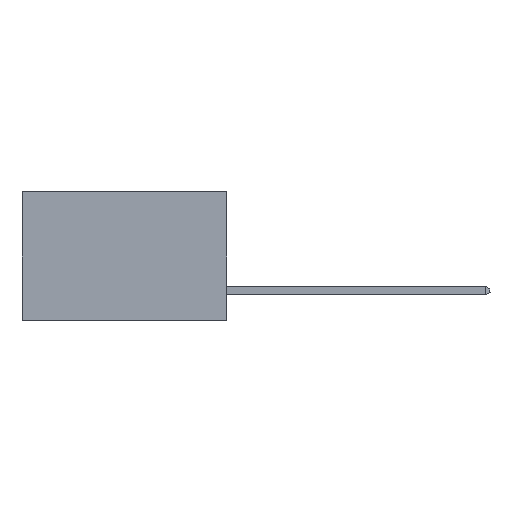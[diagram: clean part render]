
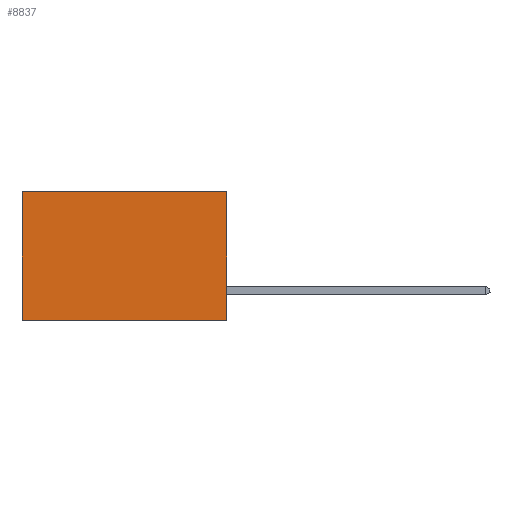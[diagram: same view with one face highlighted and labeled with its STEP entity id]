
A CAD part, left-side view. The second image highlights one B-rep face of the part: STEP entity #8837.
In plain terms, the highlighted planar face has unit normal (-1, 0, 0).
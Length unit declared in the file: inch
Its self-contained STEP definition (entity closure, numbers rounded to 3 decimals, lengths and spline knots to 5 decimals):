
#177 = VECTOR ( 'NONE', #7763, 39.37008 ) ;
#403 = LINE ( 'NONE', #4517, #2275 ) ;
#444 = VECTOR ( 'NONE', #3539, 39.37008 ) ;
#995 = CARTESIAN_POINT ( 'NONE',  ( 0.277, 0., -0.37 ) ) ;
#1180 = ORIENTED_EDGE ( 'NONE', *, *, #9418, .T. ) ;
#1226 = CARTESIAN_POINT ( 'NONE',  ( 0.277, 0., 0. ) ) ;
#1271 = DIRECTION ( 'NONE',  ( 0., 0., -1. ) ) ;
#1552 = VERTEX_POINT ( 'NONE', #6495 ) ;
#1654 = EDGE_LOOP ( 'NONE', ( #2226, #6306, #2462, #1180 ) ) ;
#1784 = EDGE_CURVE ( 'NONE', #7618, #1552, #8625, .T. ) ;
#2226 = ORIENTED_EDGE ( 'NONE', *, *, #5243, .T. ) ;
#2275 = VECTOR ( 'NONE', #1271, 39.37008 ) ;
#2458 = AXIS2_PLACEMENT_3D ( 'NONE', #3920, #3849, #3811 ) ;
#2462 = ORIENTED_EDGE ( 'NONE', *, *, #2561, .F. ) ;
#2552 = LINE ( 'NONE', #1226, #444 ) ;
#2561 = EDGE_CURVE ( 'NONE', #2669, #7618, #7122, .T. ) ;
#2669 = VERTEX_POINT ( 'NONE', #9861 ) ;
#3539 = DIRECTION ( 'NONE',  ( 0., 1., 0. ) ) ;
#3691 = FACE_OUTER_BOUND ( 'NONE', #1654, .T. ) ;
#3811 = DIRECTION ( 'NONE',  ( 0., 0., -1. ) ) ;
#3849 = DIRECTION ( 'NONE',  ( 1., 0., 0. ) ) ;
#3920 = CARTESIAN_POINT ( 'NONE',  ( 0.277, 0., -0.37 ) ) ;
#3927 = PLANE ( 'NONE',  #2458 ) ;
#3946 = DIRECTION ( 'NONE',  ( 0., 0., -1. ) ) ;
#4165 = CARTESIAN_POINT ( 'NONE',  ( 0.277, 0., -0.37 ) ) ;
#4517 = CARTESIAN_POINT ( 'NONE',  ( 0.277, 0.59, -0.37 ) ) ;
#5243 = EDGE_CURVE ( 'NONE', #8440, #1552, #403, .T. ) ;
#5698 = CARTESIAN_POINT ( 'NONE',  ( 0.277, 0.59, 0. ) ) ;
#6306 = ORIENTED_EDGE ( 'NONE', *, *, #1784, .F. ) ;
#6495 = CARTESIAN_POINT ( 'NONE',  ( 0.277, 0.59, -0.37 ) ) ;
#6873 = VECTOR ( 'NONE', #3946, 39.37008 ) ;
#6978 = CARTESIAN_POINT ( 'NONE',  ( 0.277, 0., -0.37 ) ) ;
#7122 = LINE ( 'NONE', #995, #6873 ) ;
#7618 = VERTEX_POINT ( 'NONE', #4165 ) ;
#7763 = DIRECTION ( 'NONE',  ( 0., 1., 0. ) ) ;
#8440 = VERTEX_POINT ( 'NONE', #5698 ) ;
#8625 = LINE ( 'NONE', #6978, #177 ) ;
#8837 = ADVANCED_FACE ( 'NONE', ( #3691 ), #3927, .F. ) ;
#9418 = EDGE_CURVE ( 'NONE', #2669, #8440, #2552, .T. ) ;
#9861 = CARTESIAN_POINT ( 'NONE',  ( 0.277, 0., 0. ) ) ;
